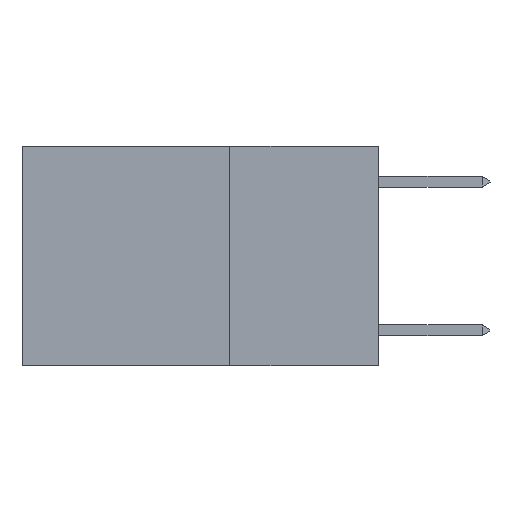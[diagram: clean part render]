
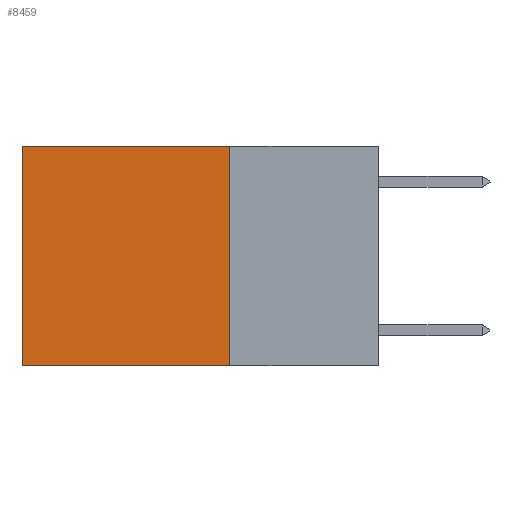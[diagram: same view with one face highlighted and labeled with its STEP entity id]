
A CAD part, left-side view. The second image highlights one B-rep face of the part: STEP entity #8459.
In plain terms, the highlighted planar face has unit normal (-1, 0, 0).
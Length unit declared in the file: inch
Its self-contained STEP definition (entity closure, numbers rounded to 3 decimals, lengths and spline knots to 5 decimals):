
#425 = CARTESIAN_POINT ( 'NONE',  ( 0.2625, 0.25, 0. ) ) ;
#1839 = VERTEX_POINT ( 'NONE', #15579 ) ;
#2898 = DIRECTION ( 'NONE',  ( 0., 1., 0. ) ) ;
#2923 = DIRECTION ( 'NONE',  ( 0., 1., 0. ) ) ;
#3220 = DIRECTION ( 'NONE',  ( 0., 0., -1. ) ) ;
#3360 = CARTESIAN_POINT ( 'NONE',  ( 0.2625, 0.6, 0. ) ) ;
#3667 = LINE ( 'NONE', #13911, #7996 ) ;
#3796 = ORIENTED_EDGE ( 'NONE', *, *, #22359, .F. ) ;
#3958 = VECTOR ( 'NONE', #2923, 39.37008 ) ;
#4089 = VECTOR ( 'NONE', #2898, 39.37008 ) ;
#5724 = EDGE_LOOP ( 'NONE', ( #21073, #3796, #17696, #9826 ) ) ;
#6318 = CARTESIAN_POINT ( 'NONE',  ( 0.2625, 0.25, 0. ) ) ;
#7996 = VECTOR ( 'NONE', #15998, 39.37008 ) ;
#8459 = ADVANCED_FACE ( 'NONE', ( #9346 ), #19523, .F. ) ;
#9346 = FACE_OUTER_BOUND ( 'NONE', #5724, .T. ) ;
#9489 = LINE ( 'NONE', #20744, #3958 ) ;
#9826 = ORIENTED_EDGE ( 'NONE', *, *, #11256, .T. ) ;
#10352 = VERTEX_POINT ( 'NONE', #3360 ) ;
#10981 = VERTEX_POINT ( 'NONE', #19751 ) ;
#11256 = EDGE_CURVE ( 'NONE', #1839, #10352, #9489, .T. ) ;
#12486 = CARTESIAN_POINT ( 'NONE',  ( 0.2625, 0.25, -0.37 ) ) ;
#12693 = LINE ( 'NONE', #14789, #4089 ) ;
#13911 = CARTESIAN_POINT ( 'NONE',  ( 0.2625, 0.6, 0. ) ) ;
#14789 = CARTESIAN_POINT ( 'NONE',  ( 0.2625, 0.25, -0.37 ) ) ;
#15058 = VERTEX_POINT ( 'NONE', #12486 ) ;
#15579 = CARTESIAN_POINT ( 'NONE',  ( 0.2625, 0.25, 0. ) ) ;
#15998 = DIRECTION ( 'NONE',  ( 0., 0., -1. ) ) ;
#16030 = EDGE_CURVE ( 'NONE', #1839, #15058, #23450, .T. ) ;
#16186 = DIRECTION ( 'NONE',  ( 0., 0., -1. ) ) ;
#16786 = DIRECTION ( 'NONE',  ( 1., 0., 0. ) ) ;
#17696 = ORIENTED_EDGE ( 'NONE', *, *, #16030, .F. ) ;
#17932 = AXIS2_PLACEMENT_3D ( 'NONE', #6318, #16786, #3220 ) ;
#19523 = PLANE ( 'NONE',  #17932 ) ;
#19751 = CARTESIAN_POINT ( 'NONE',  ( 0.2625, 0.6, -0.37 ) ) ;
#20744 = CARTESIAN_POINT ( 'NONE',  ( 0.2625, 0.25, 0. ) ) ;
#21073 = ORIENTED_EDGE ( 'NONE', *, *, #25090, .T. ) ;
#21878 = VECTOR ( 'NONE', #16186, 39.37008 ) ;
#22359 = EDGE_CURVE ( 'NONE', #15058, #10981, #12693, .T. ) ;
#23450 = LINE ( 'NONE', #425, #21878 ) ;
#25090 = EDGE_CURVE ( 'NONE', #10352, #10981, #3667, .T. ) ;
